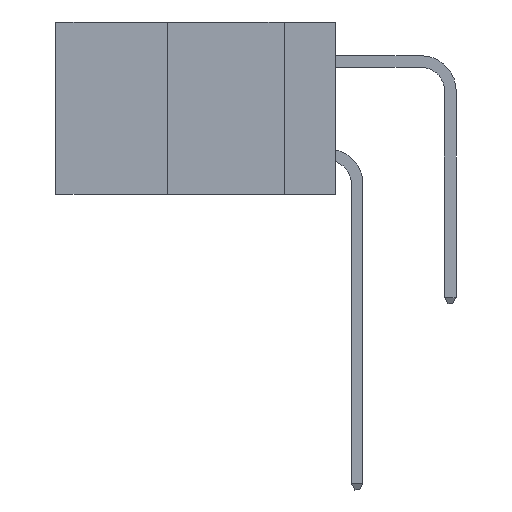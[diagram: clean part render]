
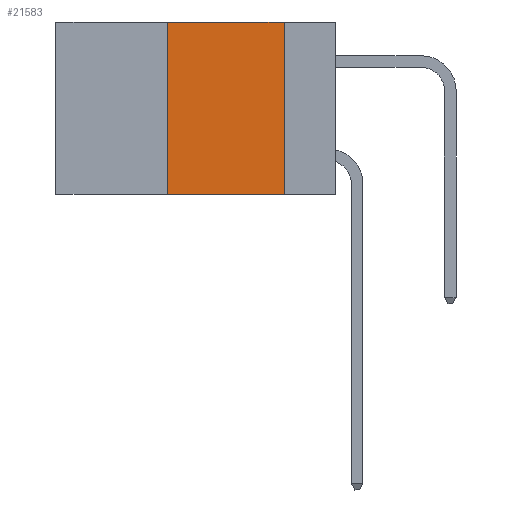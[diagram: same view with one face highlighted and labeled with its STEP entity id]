
A CAD part, left-side view. The second image highlights one B-rep face of the part: STEP entity #21583.
In plain terms, the highlighted planar face has unit normal (-1, 0, 0).
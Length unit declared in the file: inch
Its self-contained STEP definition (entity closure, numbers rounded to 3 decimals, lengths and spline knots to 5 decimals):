
#137 = FACE_OUTER_BOUND ( 'NONE', #33560, .T. ) ;
#713 = CARTESIAN_POINT ( 'NONE',  ( 0., 0.6, 0. ) ) ;
#2694 = CARTESIAN_POINT ( 'NONE',  ( 0., 0.11, 0. ) ) ;
#2718 = ORIENTED_EDGE ( 'NONE', *, *, #6984, .F. ) ;
#4388 = VERTEX_POINT ( 'NONE', #2694 ) ;
#6984 = EDGE_CURVE ( 'NONE', #4388, #17035, #32469, .T. ) ;
#7219 = VERTEX_POINT ( 'NONE', #26943 ) ;
#7566 = ORIENTED_EDGE ( 'NONE', *, *, #32962, .F. ) ;
#7642 = CARTESIAN_POINT ( 'NONE',  ( 0., 0.11, -0.37 ) ) ;
#8215 = VECTOR ( 'NONE', #34908, 39.37008 ) ;
#9288 = EDGE_CURVE ( 'NONE', #37929, #4388, #21572, .T. ) ;
#9547 = VECTOR ( 'NONE', #19918, 39.37008 ) ;
#13183 = DIRECTION ( 'NONE',  ( 0., -1., 0. ) ) ;
#15821 = ORIENTED_EDGE ( 'NONE', *, *, #25170, .T. ) ;
#16684 = CARTESIAN_POINT ( 'NONE',  ( 0., 0.6, -0.37 ) ) ;
#17035 = VERTEX_POINT ( 'NONE', #7642 ) ;
#17353 = PLANE ( 'NONE',  #25146 ) ;
#17482 = DIRECTION ( 'NONE',  ( 1., 0., 0. ) ) ;
#19918 = DIRECTION ( 'NONE',  ( 0., -1., 0. ) ) ;
#21572 = LINE ( 'NONE', #713, #28566 ) ;
#21583 = ADVANCED_FACE ( 'NONE', ( #137 ), #17353, .F. ) ;
#23044 = VECTOR ( 'NONE', #26048, 39.37008 ) ;
#25146 = AXIS2_PLACEMENT_3D ( 'NONE', #26424, #17482, #38387 ) ;
#25170 = EDGE_CURVE ( 'NONE', #7219, #17035, #33733, .T. ) ;
#26048 = DIRECTION ( 'NONE',  ( 0., 0., 1. ) ) ;
#26424 = CARTESIAN_POINT ( 'NONE',  ( 0., 0.6, 0. ) ) ;
#26943 = CARTESIAN_POINT ( 'NONE',  ( 0., 0.36, -0.37 ) ) ;
#28566 = VECTOR ( 'NONE', #13183, 39.37008 ) ;
#28729 = CARTESIAN_POINT ( 'NONE',  ( 0., 0.36, 0. ) ) ;
#28935 = CARTESIAN_POINT ( 'NONE',  ( 0., 0.11, 0. ) ) ;
#31010 = LINE ( 'NONE', #31939, #23044 ) ;
#31939 = CARTESIAN_POINT ( 'NONE',  ( 0., 0.36, 0. ) ) ;
#32469 = LINE ( 'NONE', #28935, #8215 ) ;
#32962 = EDGE_CURVE ( 'NONE', #7219, #37929, #31010, .T. ) ;
#33560 = EDGE_LOOP ( 'NONE', ( #2718, #36930, #7566, #15821 ) ) ;
#33733 = LINE ( 'NONE', #16684, #9547 ) ;
#34908 = DIRECTION ( 'NONE',  ( 0., 0., -1. ) ) ;
#36930 = ORIENTED_EDGE ( 'NONE', *, *, #9288, .F. ) ;
#37929 = VERTEX_POINT ( 'NONE', #28729 ) ;
#38387 = DIRECTION ( 'NONE',  ( 0., 0., -1. ) ) ;
